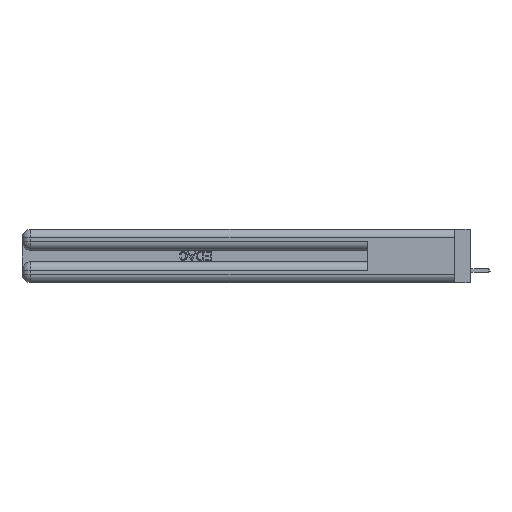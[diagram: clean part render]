
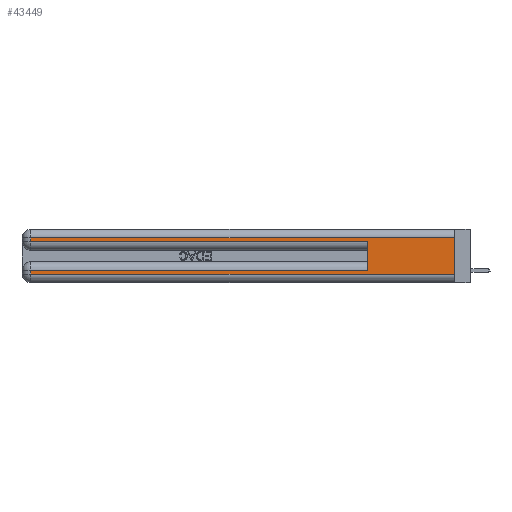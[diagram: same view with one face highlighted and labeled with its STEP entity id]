
A CAD part, left-side view. The second image highlights one B-rep face of the part: STEP entity #43449.
In plain terms, the highlighted planar face has unit normal (-1, 0, 0).
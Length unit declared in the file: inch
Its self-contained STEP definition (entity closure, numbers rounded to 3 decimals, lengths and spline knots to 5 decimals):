
#1047 = CARTESIAN_POINT ( 'NONE',  ( 0., 2.94, 0.37 ) ) ;
#1097 = CARTESIAN_POINT ( 'NONE',  ( 0., 2.94, 0.37 ) ) ;
#1155 = EDGE_CURVE ( 'NONE', #16494, #14360, #40645, .T. ) ;
#1264 = VERTEX_POINT ( 'NONE', #2625 ) ;
#2189 = ORIENTED_EDGE ( 'NONE', *, *, #1155, .T. ) ;
#2465 = ORIENTED_EDGE ( 'NONE', *, *, #28174, .T. ) ;
#2625 = CARTESIAN_POINT ( 'NONE',  ( 0., 0.6, 0.285 ) ) ;
#3238 = CARTESIAN_POINT ( 'NONE',  ( 0., 2.94, 0.085 ) ) ;
#4283 = DIRECTION ( 'NONE',  ( 0., 0., -1. ) ) ;
#4632 = DIRECTION ( 'NONE',  ( 0., 0., -1. ) ) ;
#4994 = CARTESIAN_POINT ( 'NONE',  ( 0., 0., 0.06 ) ) ;
#7248 = VERTEX_POINT ( 'NONE', #43120 ) ;
#7491 = CARTESIAN_POINT ( 'NONE',  ( 0., 0.6, 0.145 ) ) ;
#7673 = VERTEX_POINT ( 'NONE', #43067 ) ;
#7842 = CARTESIAN_POINT ( 'NONE',  ( 0., 0., 0.06 ) ) ;
#8695 = VECTOR ( 'NONE', #32993, 39.37008 ) ;
#9254 = VECTOR ( 'NONE', #43428, 39.37008 ) ;
#10129 = FACE_OUTER_BOUND ( 'NONE', #36198, .T. ) ;
#10922 = CARTESIAN_POINT ( 'NONE',  ( 0., 0., 0.37 ) ) ;
#11767 = EDGE_CURVE ( 'NONE', #17594, #13897, #15538, .T. ) ;
#12676 = LINE ( 'NONE', #14929, #41898 ) ;
#13897 = VERTEX_POINT ( 'NONE', #4994 ) ;
#14117 = EDGE_CURVE ( 'NONE', #7248, #42715, #12676, .T. ) ;
#14360 = VERTEX_POINT ( 'NONE', #16911 ) ;
#14929 = CARTESIAN_POINT ( 'NONE',  ( 0., 0., 0.085 ) ) ;
#15444 = EDGE_CURVE ( 'NONE', #7673, #13897, #34644, .T. ) ;
#15538 = LINE ( 'NONE', #15651, #16152 ) ;
#15651 = CARTESIAN_POINT ( 'NONE',  ( 0., 0., 0.37 ) ) ;
#16152 = VECTOR ( 'NONE', #20116, 39.37008 ) ;
#16494 = VERTEX_POINT ( 'NONE', #36502 ) ;
#16677 = AXIS2_PLACEMENT_3D ( 'NONE', #10922, #18016, #4283 ) ;
#16911 = CARTESIAN_POINT ( 'NONE',  ( 0., 2.94, 0.285 ) ) ;
#17594 = VERTEX_POINT ( 'NONE', #41215 ) ;
#18016 = DIRECTION ( 'NONE',  ( 1., 0., 0. ) ) ;
#18025 = VECTOR ( 'NONE', #4632, 39.37008 ) ;
#19147 = DIRECTION ( 'NONE',  ( 0., 1., 0. ) ) ;
#19575 = DIRECTION ( 'NONE',  ( 0., -1., 0. ) ) ;
#20116 = DIRECTION ( 'NONE',  ( 0., 0., -1. ) ) ;
#20794 = EDGE_CURVE ( 'NONE', #7248, #1264, #40758, .T. ) ;
#23030 = LINE ( 'NONE', #36377, #45099 ) ;
#26447 = EDGE_CURVE ( 'NONE', #14360, #1264, #23030, .T. ) ;
#26602 = EDGE_CURVE ( 'NONE', #42715, #7673, #31901, .T. ) ;
#28174 = EDGE_CURVE ( 'NONE', #17594, #16494, #41699, .T. ) ;
#31901 = LINE ( 'NONE', #1097, #9254 ) ;
#32096 = ORIENTED_EDGE ( 'NONE', *, *, #15444, .T. ) ;
#32395 = CARTESIAN_POINT ( 'NONE',  ( 0., 0., 0.31 ) ) ;
#32519 = ORIENTED_EDGE ( 'NONE', *, *, #20794, .F. ) ;
#32922 = DIRECTION ( 'NONE',  ( 0., 0., 1. ) ) ;
#32993 = DIRECTION ( 'NONE',  ( 0., -1., 0. ) ) ;
#33641 = VECTOR ( 'NONE', #32922, 39.37008 ) ;
#34644 = LINE ( 'NONE', #7842, #8695 ) ;
#36198 = EDGE_LOOP ( 'NONE', ( #44458, #2465, #2189, #36479, #32519, #40705, #41010, #32096 ) ) ;
#36218 = DIRECTION ( 'NONE',  ( 0., 1., 0. ) ) ;
#36377 = CARTESIAN_POINT ( 'NONE',  ( 0., 0., 0.285 ) ) ;
#36479 = ORIENTED_EDGE ( 'NONE', *, *, #26447, .T. ) ;
#36502 = CARTESIAN_POINT ( 'NONE',  ( 0., 2.94, 0.31 ) ) ;
#40645 = LINE ( 'NONE', #1047, #18025 ) ;
#40705 = ORIENTED_EDGE ( 'NONE', *, *, #14117, .T. ) ;
#40758 = LINE ( 'NONE', #7491, #33641 ) ;
#41010 = ORIENTED_EDGE ( 'NONE', *, *, #26602, .T. ) ;
#41215 = CARTESIAN_POINT ( 'NONE',  ( 0., 0., 0.31 ) ) ;
#41699 = LINE ( 'NONE', #32395, #43230 ) ;
#41898 = VECTOR ( 'NONE', #19147, 39.37008 ) ;
#42715 = VERTEX_POINT ( 'NONE', #3238 ) ;
#42900 = PLANE ( 'NONE',  #16677 ) ;
#43067 = CARTESIAN_POINT ( 'NONE',  ( 0., 2.94, 0.06 ) ) ;
#43120 = CARTESIAN_POINT ( 'NONE',  ( 0., 0.6, 0.085 ) ) ;
#43230 = VECTOR ( 'NONE', #36218, 39.37008 ) ;
#43428 = DIRECTION ( 'NONE',  ( 0., 0., -1. ) ) ;
#43449 = ADVANCED_FACE ( 'NONE', ( #10129 ), #42900, .F. ) ;
#44458 = ORIENTED_EDGE ( 'NONE', *, *, #11767, .F. ) ;
#45099 = VECTOR ( 'NONE', #19575, 39.37008 ) ;
